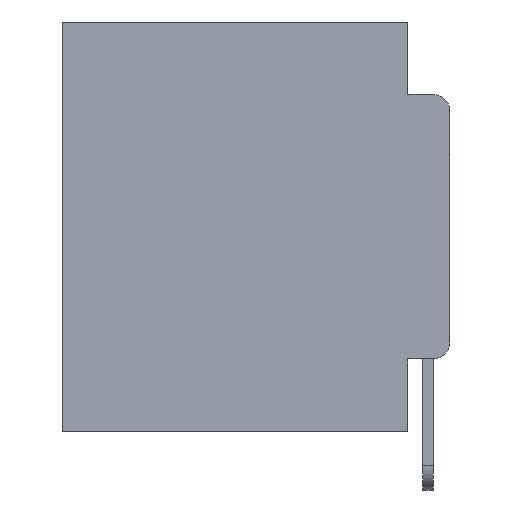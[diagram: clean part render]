
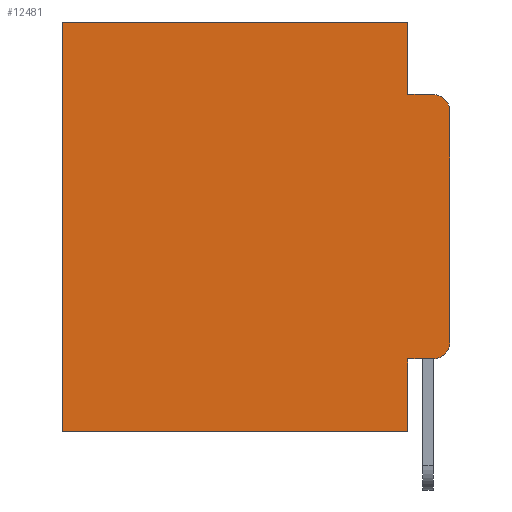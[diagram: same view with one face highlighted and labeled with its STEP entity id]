
A CAD part, left-side view. The second image highlights one B-rep face of the part: STEP entity #12481.
In plain terms, the highlighted planar face has unit normal (-1, 0, 0).
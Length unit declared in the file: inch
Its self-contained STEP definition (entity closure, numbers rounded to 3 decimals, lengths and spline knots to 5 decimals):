
#12 = EDGE_CURVE ( 'NONE', #25890, #27220, #13434, .T. ) ;
#37 = DIRECTION ( 'NONE',  ( 0., 0., -1. ) ) ;
#179 = CARTESIAN_POINT ( 'NONE',  ( 0.298, 0.051, -0.0885 ) ) ;
#265 = EDGE_CURVE ( 'NONE', #22707, #3496, #14459, .T. ) ;
#342 = ORIENTED_EDGE ( 'NONE', *, *, #10334, .F. ) ;
#605 = ORIENTED_EDGE ( 'NONE', *, *, #24042, .F. ) ;
#623 = EDGE_CURVE ( 'NONE', #4205, #11793, #15105, .T. ) ;
#2771 = CARTESIAN_POINT ( 'NONE',  ( 0.298, 0.02, -0.3915 ) ) ;
#3044 = DIRECTION ( 'NONE',  ( 0., 0., -1. ) ) ;
#3061 = VERTEX_POINT ( 'NONE', #14997 ) ;
#3155 = LINE ( 'NONE', #21806, #24385 ) ;
#3409 = LINE ( 'NONE', #18902, #20293 ) ;
#3496 = VERTEX_POINT ( 'NONE', #18264 ) ;
#3786 = CARTESIAN_POINT ( 'NONE',  ( 0.298, 0.473, 0. ) ) ;
#3856 = CARTESIAN_POINT ( 'NONE',  ( 0.298, 0.051, -0.4115 ) ) ;
#4100 = EDGE_CURVE ( 'NONE', #4205, #3061, #3155, .T. ) ;
#4205 = VERTEX_POINT ( 'NONE', #17843 ) ;
#4428 = CIRCLE ( 'NONE', #16529, 0.02 ) ;
#4570 = VECTOR ( 'NONE', #7879, 39.37008 ) ;
#4797 = ORIENTED_EDGE ( 'NONE', *, *, #7623, .T. ) ;
#4945 = AXIS2_PLACEMENT_3D ( 'NONE', #5195, #20552, #7424 ) ;
#5051 = DIRECTION ( 'NONE',  ( 0., 0., -1. ) ) ;
#5195 = CARTESIAN_POINT ( 'NONE',  ( 0.298, 0.02, -0.1085 ) ) ;
#5307 = ORIENTED_EDGE ( 'NONE', *, *, #5740, .F. ) ;
#5740 = EDGE_CURVE ( 'NONE', #16096, #25890, #3409, .T. ) ;
#6908 = AXIS2_PLACEMENT_3D ( 'NONE', #15570, #13471, #37 ) ;
#7336 = LINE ( 'NONE', #24362, #12558 ) ;
#7424 = DIRECTION ( 'NONE',  ( 0., 0., -1. ) ) ;
#7623 = EDGE_CURVE ( 'NONE', #24896, #27220, #17846, .T. ) ;
#7806 = ORIENTED_EDGE ( 'NONE', *, *, #623, .T. ) ;
#7879 = DIRECTION ( 'NONE',  ( 0., 1., 0. ) ) ;
#8296 = CARTESIAN_POINT ( 'NONE',  ( 0.298, 0.473, 0. ) ) ;
#9262 = VECTOR ( 'NONE', #27725, 39.37008 ) ;
#10334 = EDGE_CURVE ( 'NONE', #3061, #3496, #10511, .T. ) ;
#10511 = LINE ( 'NONE', #23139, #4570 ) ;
#11446 = CARTESIAN_POINT ( 'NONE',  ( 0.298, 0.051, -0.0885 ) ) ;
#11793 = VERTEX_POINT ( 'NONE', #13319 ) ;
#11798 = VECTOR ( 'NONE', #13538, 39.37008 ) ;
#11883 = EDGE_CURVE ( 'NONE', #16096, #22707, #7336, .T. ) ;
#11968 = ORIENTED_EDGE ( 'NONE', *, *, #4100, .F. ) ;
#12481 = ADVANCED_FACE ( 'NONE', ( #24345 ), #26391, .F. ) ;
#12558 = VECTOR ( 'NONE', #17982, 39.37008 ) ;
#12772 = VECTOR ( 'NONE', #16049, 39.37008 ) ;
#13319 = CARTESIAN_POINT ( 'NONE',  ( 0.298, 0.02, -0.4115 ) ) ;
#13434 = LINE ( 'NONE', #179, #12772 ) ;
#13471 = DIRECTION ( 'NONE',  ( 1., 0., 0. ) ) ;
#13538 = DIRECTION ( 'NONE',  ( 0., 0., -1. ) ) ;
#13741 = EDGE_CURVE ( 'NONE', #11793, #22739, #4428, .T. ) ;
#14459 = LINE ( 'NONE', #8296, #18191 ) ;
#14997 = CARTESIAN_POINT ( 'NONE',  ( 0.298, 0.051, -0.5 ) ) ;
#15105 = LINE ( 'NONE', #3856, #9262 ) ;
#15570 = CARTESIAN_POINT ( 'NONE',  ( 0.298, 0., 0. ) ) ;
#16049 = DIRECTION ( 'NONE',  ( 0., -1., 0. ) ) ;
#16096 = VERTEX_POINT ( 'NONE', #26429 ) ;
#16529 = AXIS2_PLACEMENT_3D ( 'NONE', #2771, #18234, #5051 ) ;
#17829 = CARTESIAN_POINT ( 'NONE',  ( 0.298, 0., 0. ) ) ;
#17843 = CARTESIAN_POINT ( 'NONE',  ( 0.298, 0.051, -0.4115 ) ) ;
#17846 = CIRCLE ( 'NONE', #4945, 0.02 ) ;
#17982 = DIRECTION ( 'NONE',  ( 0., 1., 0. ) ) ;
#18080 = ORIENTED_EDGE ( 'NONE', *, *, #11883, .T. ) ;
#18191 = VECTOR ( 'NONE', #3044, 39.37008 ) ;
#18234 = DIRECTION ( 'NONE',  ( -1., 0., 0. ) ) ;
#18264 = CARTESIAN_POINT ( 'NONE',  ( 0.298, 0.473, -0.5 ) ) ;
#18902 = CARTESIAN_POINT ( 'NONE',  ( 0.298, 0.051, 0. ) ) ;
#18948 = LINE ( 'NONE', #17829, #11798 ) ;
#19265 = CARTESIAN_POINT ( 'NONE',  ( 0.298, 0.02, -0.0885 ) ) ;
#19660 = DIRECTION ( 'NONE',  ( 0., 0., -1. ) ) ;
#20293 = VECTOR ( 'NONE', #25356, 39.37008 ) ;
#20552 = DIRECTION ( 'NONE',  ( -1., 0., 0. ) ) ;
#21806 = CARTESIAN_POINT ( 'NONE',  ( 0.298, 0.051, 0. ) ) ;
#22707 = VERTEX_POINT ( 'NONE', #3786 ) ;
#22739 = VERTEX_POINT ( 'NONE', #25751 ) ;
#23088 = ORIENTED_EDGE ( 'NONE', *, *, #13741, .T. ) ;
#23139 = CARTESIAN_POINT ( 'NONE',  ( 0.298, 0., -0.5 ) ) ;
#23372 = EDGE_LOOP ( 'NONE', ( #605, #4797, #25758, #5307, #18080, #26466, #342, #11968, #7806, #23088 ) ) ;
#24042 = EDGE_CURVE ( 'NONE', #24896, #22739, #18948, .T. ) ;
#24345 = FACE_OUTER_BOUND ( 'NONE', #23372, .T. ) ;
#24362 = CARTESIAN_POINT ( 'NONE',  ( 0.298, 0., 0. ) ) ;
#24385 = VECTOR ( 'NONE', #19660, 39.37008 ) ;
#24896 = VERTEX_POINT ( 'NONE', #27343 ) ;
#25356 = DIRECTION ( 'NONE',  ( 0., 0., -1. ) ) ;
#25751 = CARTESIAN_POINT ( 'NONE',  ( 0.298, 0., -0.3915 ) ) ;
#25758 = ORIENTED_EDGE ( 'NONE', *, *, #12, .F. ) ;
#25890 = VERTEX_POINT ( 'NONE', #11446 ) ;
#26391 = PLANE ( 'NONE',  #6908 ) ;
#26429 = CARTESIAN_POINT ( 'NONE',  ( 0.298, 0.051, 0. ) ) ;
#26466 = ORIENTED_EDGE ( 'NONE', *, *, #265, .T. ) ;
#27220 = VERTEX_POINT ( 'NONE', #19265 ) ;
#27343 = CARTESIAN_POINT ( 'NONE',  ( 0.298, 0., -0.1085 ) ) ;
#27725 = DIRECTION ( 'NONE',  ( 0., -1., 0. ) ) ;
